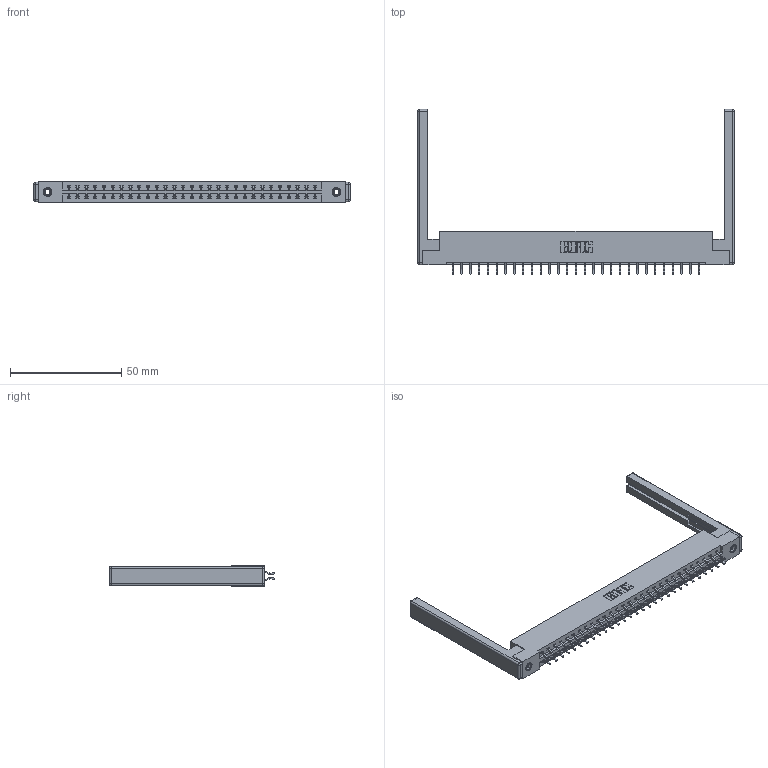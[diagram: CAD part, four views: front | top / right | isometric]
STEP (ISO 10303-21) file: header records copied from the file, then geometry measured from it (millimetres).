
FILE_DESCRIPTION (( 'STEP AP203' ), '1' );
FILE_NAME ('337-058-556-268.STEP', '2019-10-09T19:59:11', ( '' ), ( '' ), 'SwSTEP 2.0', 'SolidWorks 2016', '' );
FILE_SCHEMA (( 'CONFIG_CONTROL_DESIGN' ));
Length unit declared in the file: inch
Products named in the file (5): 337 Part_Flush Mounting Lugs - 0.156 Dia-TI; 307-220-068; 345-250-001_345-250-001-102; 337-058-556-268; 345-292-001_556 Tail
Assembly tree (63 placements, depth 2):
  337-058-556-268
    337 Part_Flush Mounting Lugs - 0.156 Dia-TI
    345-292-001_556 Tail  x58
    345-250-001_345-250-001-102  x2
    307-220-068  x2
Bounding box: 142.34 x 74.31 x 9.4 mm (x, y, z)
Volume: 19210.5 mm3; surface area: 20607.4 mm2
Topology: 63 solids, 63 shells, 3748 faces, 11083 edges, 7290 vertices
Faces by surface type: plane 2594, cylinder 1130, cone 12, sphere 8, torus 4
Entity records: 27146 total; most frequent: CARTESIAN_POINT 4563, ORIENTED_EDGE 4476, DIRECTION 3964, EDGE_CURVE 2238, VECTOR 2052, LINE 2052, VERTEX_POINT 1482, AXIS2_PLACEMENT_3D 956
